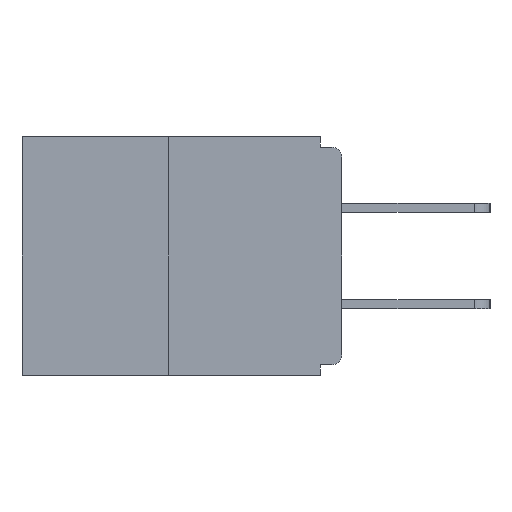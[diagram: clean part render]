
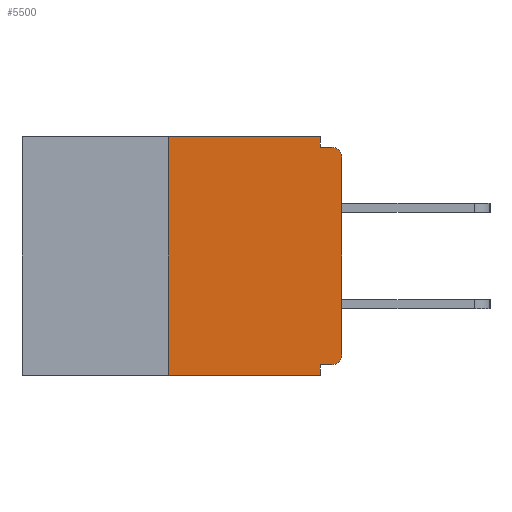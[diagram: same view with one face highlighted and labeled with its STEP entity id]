
A CAD part, left-side view. The second image highlights one B-rep face of the part: STEP entity #5500.
In plain terms, the highlighted planar face has unit normal (-1, 0, 0).
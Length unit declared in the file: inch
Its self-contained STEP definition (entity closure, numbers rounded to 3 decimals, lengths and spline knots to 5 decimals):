
#347 = VERTEX_POINT ( 'NONE', #9906 ) ;
#468 = VECTOR ( 'NONE', #4375, 39.37008 ) ;
#503 = CARTESIAN_POINT ( 'NONE',  ( 0., 0.46, 0. ) ) ;
#713 = DIRECTION ( 'NONE',  ( 0., 1., 0. ) ) ;
#737 = DIRECTION ( 'NONE',  ( 0., 0., -1. ) ) ;
#954 = CARTESIAN_POINT ( 'NONE',  ( 0., 0., -0.328 ) ) ;
#1345 = VECTOR ( 'NONE', #713, 39.37008 ) ;
#1408 = ORIENTED_EDGE ( 'NONE', *, *, #7568, .F. ) ;
#1585 = CARTESIAN_POINT ( 'NONE',  ( 0., 0.015, -0.015 ) ) ;
#1679 = CARTESIAN_POINT ( 'NONE',  ( 0., 0.015, -0.313 ) ) ;
#1733 = AXIS2_PLACEMENT_3D ( 'NONE', #2040, #7788, #1979 ) ;
#1790 = CARTESIAN_POINT ( 'NONE',  ( 0., 0., -0.03 ) ) ;
#1810 = LINE ( 'NONE', #8408, #3606 ) ;
#1837 = CARTESIAN_POINT ( 'NONE',  ( 0., 0.031, -0.328 ) ) ;
#1913 = VERTEX_POINT ( 'NONE', #1585 ) ;
#1921 = DIRECTION ( 'NONE',  ( 0., -1., 0. ) ) ;
#1940 = ORIENTED_EDGE ( 'NONE', *, *, #2632, .F. ) ;
#1979 = DIRECTION ( 'NONE',  ( 0., 0., -1. ) ) ;
#2040 = CARTESIAN_POINT ( 'NONE',  ( 0., 0.015, -0.03 ) ) ;
#2158 = VERTEX_POINT ( 'NONE', #8221 ) ;
#2194 = VECTOR ( 'NONE', #5294, 39.37008 ) ;
#2217 = DIRECTION ( 'NONE',  ( 1., 0., 0. ) ) ;
#2396 = VECTOR ( 'NONE', #4350, 39.37008 ) ;
#2632 = EDGE_CURVE ( 'NONE', #347, #3206, #1810, .T. ) ;
#3007 = CARTESIAN_POINT ( 'NONE',  ( 0., 0.46, -0.343 ) ) ;
#3206 = VERTEX_POINT ( 'NONE', #4783 ) ;
#3410 = VERTEX_POINT ( 'NONE', #1837 ) ;
#3572 = AXIS2_PLACEMENT_3D ( 'NONE', #1679, #5416, #737 ) ;
#3606 = VECTOR ( 'NONE', #1921, 39.37008 ) ;
#3870 = LINE ( 'NONE', #3007, #7145 ) ;
#3910 = VERTEX_POINT ( 'NONE', #8120 ) ;
#3928 = DIRECTION ( 'NONE',  ( 0., 0., -1. ) ) ;
#4041 = FACE_OUTER_BOUND ( 'NONE', #7277, .T. ) ;
#4154 = LINE ( 'NONE', #11886, #2396 ) ;
#4173 = LINE ( 'NONE', #11842, #468 ) ;
#4350 = DIRECTION ( 'NONE',  ( 0., 0., 1. ) ) ;
#4375 = DIRECTION ( 'NONE',  ( 0., 0., 1. ) ) ;
#4423 = VERTEX_POINT ( 'NONE', #10219 ) ;
#4519 = ORIENTED_EDGE ( 'NONE', *, *, #7203, .F. ) ;
#4742 = LINE ( 'NONE', #11520, #10557 ) ;
#4783 = CARTESIAN_POINT ( 'NONE',  ( 0., 0.031, 0. ) ) ;
#5103 = ORIENTED_EDGE ( 'NONE', *, *, #9003, .T. ) ;
#5294 = DIRECTION ( 'NONE',  ( 0., 0., -1. ) ) ;
#5326 = LINE ( 'NONE', #7285, #5914 ) ;
#5416 = DIRECTION ( 'NONE',  ( -1., 0., 0. ) ) ;
#5500 = ADVANCED_FACE ( 'NONE', ( #4041 ), #10672, .F. ) ;
#5557 = CIRCLE ( 'NONE', #3572, 0.015 ) ;
#5821 = CIRCLE ( 'NONE', #1733, 0.015 ) ;
#5914 = VECTOR ( 'NONE', #9366, 39.37008 ) ;
#6089 = LINE ( 'NONE', #8083, #2194 ) ;
#6226 = EDGE_CURVE ( 'NONE', #4423, #2158, #5557, .T. ) ;
#6725 = ORIENTED_EDGE ( 'NONE', *, *, #10362, .F. ) ;
#7145 = VECTOR ( 'NONE', #9748, 39.37008 ) ;
#7203 = EDGE_CURVE ( 'NONE', #11205, #1913, #5326, .T. ) ;
#7277 = EDGE_LOOP ( 'NONE', ( #1940, #10408, #8483, #10056, #6725, #9937, #7429, #5103, #4519, #1408 ) ) ;
#7285 = CARTESIAN_POINT ( 'NONE',  ( 0., 0., -0.015 ) ) ;
#7364 = EDGE_CURVE ( 'NONE', #10122, #3910, #3870, .T. ) ;
#7429 = ORIENTED_EDGE ( 'NONE', *, *, #8865, .T. ) ;
#7467 = LINE ( 'NONE', #954, #1345 ) ;
#7568 = EDGE_CURVE ( 'NONE', #3206, #11205, #6089, .T. ) ;
#7788 = DIRECTION ( 'NONE',  ( -1., 0., 0. ) ) ;
#7941 = EDGE_CURVE ( 'NONE', #10122, #347, #4154, .T. ) ;
#8083 = CARTESIAN_POINT ( 'NONE',  ( 0., 0.031, 0. ) ) ;
#8120 = CARTESIAN_POINT ( 'NONE',  ( 0., 0.031, -0.343 ) ) ;
#8221 = CARTESIAN_POINT ( 'NONE',  ( 0., 0., -0.313 ) ) ;
#8408 = CARTESIAN_POINT ( 'NONE',  ( 0., 0.46, 0. ) ) ;
#8483 = ORIENTED_EDGE ( 'NONE', *, *, #7364, .T. ) ;
#8865 = EDGE_CURVE ( 'NONE', #2158, #9549, #4173, .T. ) ;
#9003 = EDGE_CURVE ( 'NONE', #9549, #1913, #5821, .T. ) ;
#9056 = EDGE_CURVE ( 'NONE', #3410, #3910, #4742, .T. ) ;
#9366 = DIRECTION ( 'NONE',  ( 0., -1., 0. ) ) ;
#9549 = VERTEX_POINT ( 'NONE', #1790 ) ;
#9748 = DIRECTION ( 'NONE',  ( 0., -1., 0. ) ) ;
#9889 = AXIS2_PLACEMENT_3D ( 'NONE', #503, #2217, #10799 ) ;
#9906 = CARTESIAN_POINT ( 'NONE',  ( 0., 0.25, 0. ) ) ;
#9937 = ORIENTED_EDGE ( 'NONE', *, *, #6226, .T. ) ;
#10056 = ORIENTED_EDGE ( 'NONE', *, *, #9056, .F. ) ;
#10122 = VERTEX_POINT ( 'NONE', #10814 ) ;
#10219 = CARTESIAN_POINT ( 'NONE',  ( 0., 0.015, -0.328 ) ) ;
#10362 = EDGE_CURVE ( 'NONE', #4423, #3410, #7467, .T. ) ;
#10408 = ORIENTED_EDGE ( 'NONE', *, *, #7941, .F. ) ;
#10447 = CARTESIAN_POINT ( 'NONE',  ( 0., 0.031, -0.015 ) ) ;
#10557 = VECTOR ( 'NONE', #3928, 39.37008 ) ;
#10672 = PLANE ( 'NONE',  #9889 ) ;
#10799 = DIRECTION ( 'NONE',  ( 0., 0., -1. ) ) ;
#10814 = CARTESIAN_POINT ( 'NONE',  ( 0., 0.25, -0.343 ) ) ;
#11205 = VERTEX_POINT ( 'NONE', #10447 ) ;
#11520 = CARTESIAN_POINT ( 'NONE',  ( 0., 0.031, -0.343 ) ) ;
#11842 = CARTESIAN_POINT ( 'NONE',  ( 0., 0., 0. ) ) ;
#11886 = CARTESIAN_POINT ( 'NONE',  ( 0., 0.25, 0. ) ) ;
